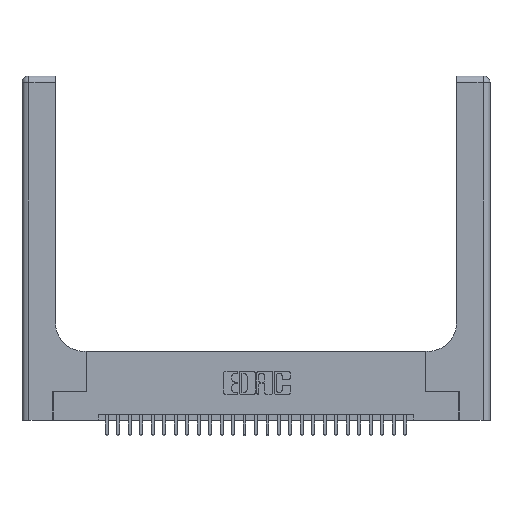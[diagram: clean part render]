
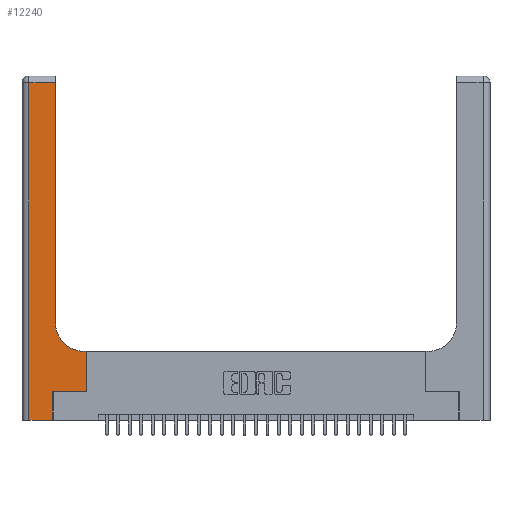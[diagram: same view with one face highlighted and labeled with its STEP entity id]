
A CAD part, top view. The second image highlights one B-rep face of the part: STEP entity #12240.
In plain terms, the highlighted planar face has unit normal (0, 0, 1).
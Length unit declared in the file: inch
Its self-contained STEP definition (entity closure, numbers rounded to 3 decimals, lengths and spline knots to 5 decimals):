
#667 = CARTESIAN_POINT ( 'NONE',  ( 0.5415, 0.85, 0.37 ) ) ;
#1585 = LINE ( 'NONE', #28019, #5706 ) ;
#1761 = LINE ( 'NONE', #20023, #27160 ) ;
#2217 = CARTESIAN_POINT ( 'NONE',  ( 0.5415, 0.6, 0.37 ) ) ;
#2678 = CARTESIAN_POINT ( 'NONE',  ( 0.5585, 0.25, 0.37 ) ) ;
#3142 = LINE ( 'NONE', #12820, #14855 ) ;
#3265 = DIRECTION ( 'NONE',  ( 0., 0., -1. ) ) ;
#3629 = VERTEX_POINT ( 'NONE', #14763 ) ;
#4673 = VERTEX_POINT ( 'NONE', #2678 ) ;
#5121 = FACE_OUTER_BOUND ( 'NONE', #22240, .T. ) ;
#5648 = AXIS2_PLACEMENT_3D ( 'NONE', #9810, #3265, #14328 ) ;
#5651 = CARTESIAN_POINT ( 'NONE',  ( 0., 0., 0.37 ) ) ;
#5706 = VECTOR ( 'NONE', #12489, 39.37008 ) ;
#5835 = EDGE_CURVE ( 'NONE', #4673, #12126, #1761, .T. ) ;
#5995 = VECTOR ( 'NONE', #26285, 39.37008 ) ;
#5996 = VECTOR ( 'NONE', #6561, 39.37008 ) ;
#6121 = ORIENTED_EDGE ( 'NONE', *, *, #8005, .T. ) ;
#6561 = DIRECTION ( 'NONE',  ( 0., -1., 0. ) ) ;
#6819 = DIRECTION ( 'NONE',  ( 0., 1., 0. ) ) ;
#7865 = LINE ( 'NONE', #18954, #26715 ) ;
#8005 = EDGE_CURVE ( 'NONE', #14003, #25524, #7865, .T. ) ;
#8026 = CARTESIAN_POINT ( 'NONE',  ( 0.06, 2.94, 0.37 ) ) ;
#8028 = VERTEX_POINT ( 'NONE', #8026 ) ;
#8145 = DIRECTION ( 'NONE',  ( 1., 0., 0. ) ) ;
#8590 = DIRECTION ( 'NONE',  ( 1., 0., 0. ) ) ;
#8967 = CIRCLE ( 'NONE', #10525, 0.25 ) ;
#9187 = ORIENTED_EDGE ( 'NONE', *, *, #10027, .T. ) ;
#9772 = ORIENTED_EDGE ( 'NONE', *, *, #26917, .T. ) ;
#9810 = CARTESIAN_POINT ( 'NONE',  ( 0., 3., 0.37 ) ) ;
#10027 = EDGE_CURVE ( 'NONE', #25524, #4673, #3142, .T. ) ;
#10525 = AXIS2_PLACEMENT_3D ( 'NONE', #667, #22951, #26962 ) ;
#11938 = VECTOR ( 'NONE', #27432, 39.37008 ) ;
#12126 = VERTEX_POINT ( 'NONE', #24109 ) ;
#12240 = ADVANCED_FACE ( 'NONE', ( #5121 ), #22946, .F. ) ;
#12489 = DIRECTION ( 'NONE',  ( -1., 0., 0. ) ) ;
#12820 = CARTESIAN_POINT ( 'NONE',  ( 0.269, 0.25, 0.37 ) ) ;
#12981 = CARTESIAN_POINT ( 'NONE',  ( 0., 2.94, 0.37 ) ) ;
#13023 = EDGE_CURVE ( 'NONE', #16113, #21545, #20200, .T. ) ;
#13640 = CARTESIAN_POINT ( 'NONE',  ( 0.2915, 2.94, 0.37 ) ) ;
#13756 = EDGE_CURVE ( 'NONE', #12126, #27743, #1585, .T. ) ;
#14003 = VERTEX_POINT ( 'NONE', #26551 ) ;
#14305 = CARTESIAN_POINT ( 'NONE',  ( 0.2915, 3., 0.37 ) ) ;
#14328 = DIRECTION ( 'NONE',  ( -1., 0., 0. ) ) ;
#14763 = CARTESIAN_POINT ( 'NONE',  ( 0.06, 0., 0.37 ) ) ;
#14855 = VECTOR ( 'NONE', #8590, 39.37008 ) ;
#16058 = EDGE_CURVE ( 'NONE', #3629, #14003, #24919, .T. ) ;
#16113 = VERTEX_POINT ( 'NONE', #21591 ) ;
#16779 = EDGE_CURVE ( 'NONE', #21545, #8028, #17685, .T. ) ;
#17685 = LINE ( 'NONE', #12981, #5995 ) ;
#18954 = CARTESIAN_POINT ( 'NONE',  ( 0.269, 0., 0.37 ) ) ;
#19101 = VECTOR ( 'NONE', #8145, 39.37008 ) ;
#20023 = CARTESIAN_POINT ( 'NONE',  ( 0.5585, 0.25, 0.37 ) ) ;
#20200 = LINE ( 'NONE', #14305, #11938 ) ;
#21150 = LINE ( 'NONE', #26331, #5996 ) ;
#21349 = ORIENTED_EDGE ( 'NONE', *, *, #13023, .T. ) ;
#21545 = VERTEX_POINT ( 'NONE', #13640 ) ;
#21591 = CARTESIAN_POINT ( 'NONE',  ( 0.2915, 0.85, 0.37 ) ) ;
#22240 = EDGE_LOOP ( 'NONE', ( #21349, #28321, #9772, #27913, #6121, #9187, #26913, #27814, #24453 ) ) ;
#22946 = PLANE ( 'NONE',  #5648 ) ;
#22951 = DIRECTION ( 'NONE',  ( 0., 0., -1. ) ) ;
#23168 = EDGE_CURVE ( 'NONE', #27743, #16113, #8967, .T. ) ;
#24109 = CARTESIAN_POINT ( 'NONE',  ( 0.5585, 0.6, 0.37 ) ) ;
#24453 = ORIENTED_EDGE ( 'NONE', *, *, #23168, .T. ) ;
#24919 = LINE ( 'NONE', #5651, #19101 ) ;
#25465 = DIRECTION ( 'NONE',  ( 0., 1., 0. ) ) ;
#25524 = VERTEX_POINT ( 'NONE', #27856 ) ;
#26285 = DIRECTION ( 'NONE',  ( -1., 0., 0. ) ) ;
#26331 = CARTESIAN_POINT ( 'NONE',  ( 0.06, 3., 0.37 ) ) ;
#26551 = CARTESIAN_POINT ( 'NONE',  ( 0.269, 0., 0.37 ) ) ;
#26715 = VECTOR ( 'NONE', #25465, 39.37008 ) ;
#26913 = ORIENTED_EDGE ( 'NONE', *, *, #5835, .T. ) ;
#26917 = EDGE_CURVE ( 'NONE', #8028, #3629, #21150, .T. ) ;
#26962 = DIRECTION ( 'NONE',  ( 1., 0., 0. ) ) ;
#27160 = VECTOR ( 'NONE', #6819, 39.37008 ) ;
#27432 = DIRECTION ( 'NONE',  ( 0., 1., 0. ) ) ;
#27743 = VERTEX_POINT ( 'NONE', #2217 ) ;
#27814 = ORIENTED_EDGE ( 'NONE', *, *, #13756, .T. ) ;
#27856 = CARTESIAN_POINT ( 'NONE',  ( 0.269, 0.25, 0.37 ) ) ;
#27913 = ORIENTED_EDGE ( 'NONE', *, *, #16058, .T. ) ;
#28019 = CARTESIAN_POINT ( 'NONE',  ( 0.2915, 0.6, 0.37 ) ) ;
#28321 = ORIENTED_EDGE ( 'NONE', *, *, #16779, .T. ) ;
